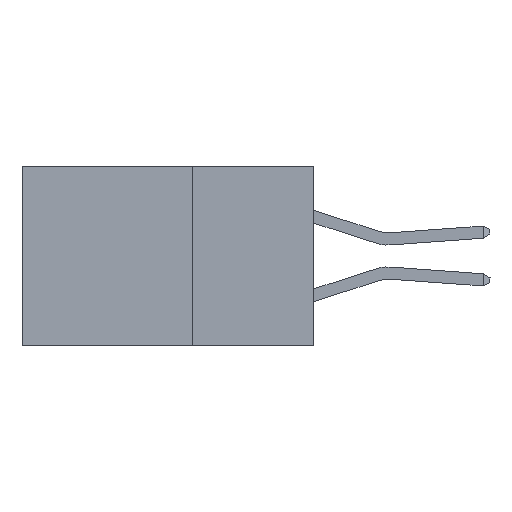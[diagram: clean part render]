
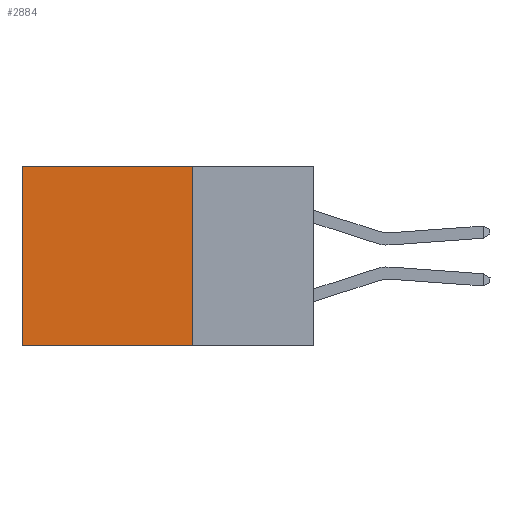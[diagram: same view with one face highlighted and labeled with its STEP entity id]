
A CAD part, left-side view. The second image highlights one B-rep face of the part: STEP entity #2884.
In plain terms, the highlighted planar face has unit normal (-1, 0, 0).
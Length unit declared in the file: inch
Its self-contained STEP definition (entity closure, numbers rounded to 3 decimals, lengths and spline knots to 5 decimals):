
#129 = DIRECTION ( 'NONE',  ( 1., 0., 0. ) ) ;
#154 = DIRECTION ( 'NONE',  ( 0., 1., 0. ) ) ;
#609 = DIRECTION ( 'NONE',  ( 0., 1., 0. ) ) ;
#622 = VECTOR ( 'NONE', #609, 39.37008 ) ;
#849 = VECTOR ( 'NONE', #3200, 39.37008 ) ;
#1393 = VERTEX_POINT ( 'NONE', #12987 ) ;
#1483 = DIRECTION ( 'NONE',  ( 0., 0., -1. ) ) ;
#1901 = VERTEX_POINT ( 'NONE', #7535 ) ;
#2656 = ORIENTED_EDGE ( 'NONE', *, *, #13317, .F. ) ;
#2884 = ADVANCED_FACE ( 'NONE', ( #6307 ), #12188, .F. ) ;
#3200 = DIRECTION ( 'NONE',  ( 0., 0., -1. ) ) ;
#5064 = CARTESIAN_POINT ( 'NONE',  ( 0.2875, 0.25, -0.37 ) ) ;
#5071 = LINE ( 'NONE', #11290, #9695 ) ;
#5086 = ORIENTED_EDGE ( 'NONE', *, *, #11329, .T. ) ;
#5572 = ORIENTED_EDGE ( 'NONE', *, *, #10234, .T. ) ;
#6307 = FACE_OUTER_BOUND ( 'NONE', #13515, .T. ) ;
#6840 = CARTESIAN_POINT ( 'NONE',  ( 0.2875, 0.25, 0. ) ) ;
#7535 = CARTESIAN_POINT ( 'NONE',  ( 0.2875, 0.6, -0.37 ) ) ;
#7539 = EDGE_CURVE ( 'NONE', #12409, #1901, #12807, .T. ) ;
#7684 = CARTESIAN_POINT ( 'NONE',  ( 0.2875, 0.25, 0. ) ) ;
#7708 = LINE ( 'NONE', #13301, #10473 ) ;
#8390 = ORIENTED_EDGE ( 'NONE', *, *, #7539, .F. ) ;
#8483 = CARTESIAN_POINT ( 'NONE',  ( 0.2875, 0.25, 0. ) ) ;
#8692 = AXIS2_PLACEMENT_3D ( 'NONE', #6840, #129, #13364 ) ;
#9695 = VECTOR ( 'NONE', #1483, 39.37008 ) ;
#10234 = EDGE_CURVE ( 'NONE', #11576, #1393, #7708, .T. ) ;
#10473 = VECTOR ( 'NONE', #154, 39.37008 ) ;
#11290 = CARTESIAN_POINT ( 'NONE',  ( 0.2875, 0.6, 0. ) ) ;
#11329 = EDGE_CURVE ( 'NONE', #1393, #1901, #5071, .T. ) ;
#11576 = VERTEX_POINT ( 'NONE', #8483 ) ;
#11651 = CARTESIAN_POINT ( 'NONE',  ( 0.2875, 0.25, -0.37 ) ) ;
#12188 = PLANE ( 'NONE',  #8692 ) ;
#12409 = VERTEX_POINT ( 'NONE', #11651 ) ;
#12807 = LINE ( 'NONE', #5064, #622 ) ;
#12987 = CARTESIAN_POINT ( 'NONE',  ( 0.2875, 0.6, 0. ) ) ;
#13208 = LINE ( 'NONE', #7684, #849 ) ;
#13301 = CARTESIAN_POINT ( 'NONE',  ( 0.2875, 0.25, 0. ) ) ;
#13317 = EDGE_CURVE ( 'NONE', #11576, #12409, #13208, .T. ) ;
#13364 = DIRECTION ( 'NONE',  ( 0., 0., -1. ) ) ;
#13515 = EDGE_LOOP ( 'NONE', ( #5086, #8390, #2656, #5572 ) ) ;
